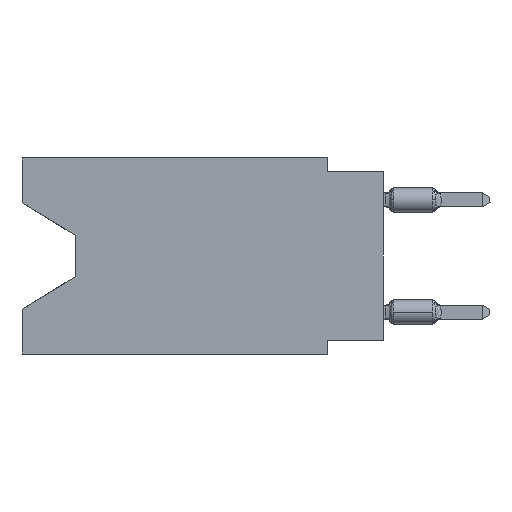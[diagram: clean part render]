
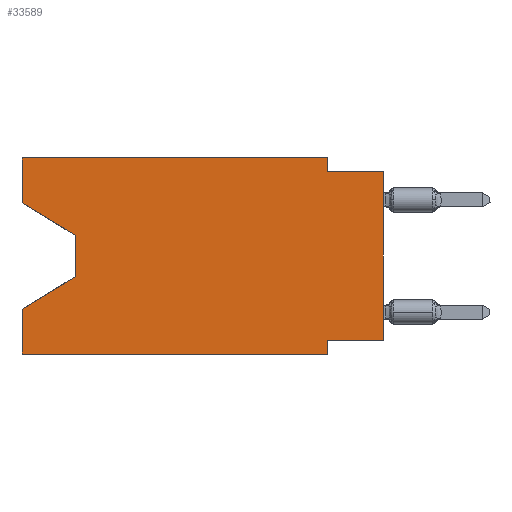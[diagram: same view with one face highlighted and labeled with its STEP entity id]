
A CAD part, left-side view. The second image highlights one B-rep face of the part: STEP entity #33589.
In plain terms, the highlighted planar face has unit normal (-1, 0, 0).
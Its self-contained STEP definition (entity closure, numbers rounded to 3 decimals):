
#683 = DIRECTION ( 'NONE',  ( 0., 0., 1. ) ) ;
#956 = CARTESIAN_POINT ( 'NONE',  ( 0., 2.54, -8.255 ) ) ;
#1462 = DIRECTION ( 'NONE',  ( 0., -0.855, -0.519 ) ) ;
#2571 = ORIENTED_EDGE ( 'NONE', *, *, #12025, .F. ) ;
#3016 = CARTESIAN_POINT ( 'NONE',  ( 0., 13.97, -5.385 ) ) ;
#3357 = EDGE_CURVE ( 'NONE', #35843, #12292, #34434, .T. ) ;
#3994 = LINE ( 'NONE', #14926, #8670 ) ;
#4325 = ORIENTED_EDGE ( 'NONE', *, *, #32457, .F. ) ;
#4568 = ORIENTED_EDGE ( 'NONE', *, *, #39529, .F. ) ;
#4733 = CARTESIAN_POINT ( 'NONE',  ( 0., 16.383, -6.852 ) ) ;
#4931 = VECTOR ( 'NONE', #32310, 1000. ) ;
#5075 = ORIENTED_EDGE ( 'NONE', *, *, #31634, .F. ) ;
#5593 = VERTEX_POINT ( 'NONE', #46168 ) ;
#6111 = LINE ( 'NONE', #3016, #12749 ) ;
#7310 = DIRECTION ( 'NONE',  ( 0., 1., 0. ) ) ;
#8323 = CARTESIAN_POINT ( 'NONE',  ( 0., 13.97, -3.505 ) ) ;
#8378 = DIRECTION ( 'NONE',  ( 0., -1., 0. ) ) ;
#8670 = VECTOR ( 'NONE', #683, 1000. ) ;
#8930 = EDGE_CURVE ( 'NONE', #29006, #25882, #6111, .T. ) ;
#9010 = VECTOR ( 'NONE', #12647, 1000. ) ;
#11980 = DIRECTION ( 'NONE',  ( 0., -1., 0. ) ) ;
#12025 = EDGE_CURVE ( 'NONE', #16454, #5593, #29225, .T. ) ;
#12292 = VERTEX_POINT ( 'NONE', #23740 ) ;
#12314 = CARTESIAN_POINT ( 'NONE',  ( 0., 13.97, -5.385 ) ) ;
#12479 = CARTESIAN_POINT ( 'NONE',  ( 0., 16.383, 0. ) ) ;
#12647 = DIRECTION ( 'NONE',  ( 0., 0., -1. ) ) ;
#12749 = VECTOR ( 'NONE', #20538, 1000. ) ;
#13089 = CARTESIAN_POINT ( 'NONE',  ( 0., 0., -8.255 ) ) ;
#13542 = EDGE_CURVE ( 'NONE', #32646, #16454, #29089, .T. ) ;
#13664 = ORIENTED_EDGE ( 'NONE', *, *, #8930, .T. ) ;
#14042 = VECTOR ( 'NONE', #8378, 1000. ) ;
#14347 = CARTESIAN_POINT ( 'NONE',  ( 0., 2.54, -8.89 ) ) ;
#14559 = EDGE_CURVE ( 'NONE', #20537, #5593, #26353, .T. ) ;
#14644 = LINE ( 'NONE', #29059, #44240 ) ;
#14926 = CARTESIAN_POINT ( 'NONE',  ( 0., 16.383, 0. ) ) ;
#15206 = LINE ( 'NONE', #8323, #23613 ) ;
#16454 = VERTEX_POINT ( 'NONE', #956 ) ;
#17372 = CARTESIAN_POINT ( 'NONE',  ( 0., 0., -8.255 ) ) ;
#17870 = LINE ( 'NONE', #40113, #4931 ) ;
#17963 = CARTESIAN_POINT ( 'NONE',  ( 0., 16.383, 0. ) ) ;
#19497 = CARTESIAN_POINT ( 'NONE',  ( 0., 2.54, 0. ) ) ;
#20196 = VECTOR ( 'NONE', #40579, 1000. ) ;
#20537 = VERTEX_POINT ( 'NONE', #46764 ) ;
#20538 = DIRECTION ( 'NONE',  ( 0., 0.855, -0.519 ) ) ;
#21754 = CARTESIAN_POINT ( 'NONE',  ( 0., 13.97, -3.505 ) ) ;
#22084 = ORIENTED_EDGE ( 'NONE', *, *, #40878, .F. ) ;
#22279 = LINE ( 'NONE', #22744, #36389 ) ;
#22744 = CARTESIAN_POINT ( 'NONE',  ( 0., 16.383, 0. ) ) ;
#23613 = VECTOR ( 'NONE', #34120, 1000. ) ;
#23740 = CARTESIAN_POINT ( 'NONE',  ( 0., 2.54, -0.635 ) ) ;
#24313 = ORIENTED_EDGE ( 'NONE', *, *, #13542, .F. ) ;
#25882 = VERTEX_POINT ( 'NONE', #4733 ) ;
#26216 = DIRECTION ( 'NONE',  ( 0., 0., -1. ) ) ;
#26319 = CARTESIAN_POINT ( 'NONE',  ( 0., 16.383, -2.038 ) ) ;
#26353 = LINE ( 'NONE', #40806, #14042 ) ;
#26596 = EDGE_LOOP ( 'NONE', ( #43565, #34264, #13664, #5075, #45835, #2571, #24313, #46116, #22084, #37100, #4325, #4568 ) ) ;
#27401 = VERTEX_POINT ( 'NONE', #21754 ) ;
#28870 = VERTEX_POINT ( 'NONE', #30532 ) ;
#29006 = VERTEX_POINT ( 'NONE', #12314 ) ;
#29059 = CARTESIAN_POINT ( 'NONE',  ( 0., 0., 0. ) ) ;
#29089 = LINE ( 'NONE', #13089, #41152 ) ;
#29225 = LINE ( 'NONE', #14347, #20196 ) ;
#30532 = CARTESIAN_POINT ( 'NONE',  ( 0., 16.383, -2.038 ) ) ;
#31600 = CARTESIAN_POINT ( 'NONE',  ( 0., 0., -0.635 ) ) ;
#31634 = EDGE_CURVE ( 'NONE', #20537, #25882, #3994, .T. ) ;
#32310 = DIRECTION ( 'NONE',  ( 0., -1., 0. ) ) ;
#32457 = EDGE_CURVE ( 'NONE', #37434, #35843, #17870, .T. ) ;
#32646 = VERTEX_POINT ( 'NONE', #17372 ) ;
#33589 = ADVANCED_FACE ( 'NONE', ( #43758 ), #44425, .F. ) ;
#33707 = CARTESIAN_POINT ( 'NONE',  ( 0., 2.54, 0. ) ) ;
#34120 = DIRECTION ( 'NONE',  ( 0., 0., -1. ) ) ;
#34264 = ORIENTED_EDGE ( 'NONE', *, *, #41236, .T. ) ;
#34434 = LINE ( 'NONE', #19497, #9010 ) ;
#35843 = VERTEX_POINT ( 'NONE', #33707 ) ;
#36389 = VECTOR ( 'NONE', #36725, 1000. ) ;
#36725 = DIRECTION ( 'NONE',  ( 0., 0., 1. ) ) ;
#36986 = EDGE_CURVE ( 'NONE', #28870, #27401, #41457, .T. ) ;
#37081 = LINE ( 'NONE', #44391, #45505 ) ;
#37100 = ORIENTED_EDGE ( 'NONE', *, *, #3357, .F. ) ;
#37434 = VERTEX_POINT ( 'NONE', #12479 ) ;
#38756 = VECTOR ( 'NONE', #1462, 1000. ) ;
#39529 = EDGE_CURVE ( 'NONE', #28870, #37434, #22279, .T. ) ;
#40113 = CARTESIAN_POINT ( 'NONE',  ( 0., 16.383, 0. ) ) ;
#40440 = DIRECTION ( 'NONE',  ( 1., 0., 0. ) ) ;
#40579 = DIRECTION ( 'NONE',  ( 0., 0., -1. ) ) ;
#40806 = CARTESIAN_POINT ( 'NONE',  ( 0., 16.383, -8.89 ) ) ;
#40878 = EDGE_CURVE ( 'NONE', #12292, #43611, #37081, .T. ) ;
#41152 = VECTOR ( 'NONE', #7310, 1000. ) ;
#41194 = AXIS2_PLACEMENT_3D ( 'NONE', #17963, #40440, #26216 ) ;
#41236 = EDGE_CURVE ( 'NONE', #27401, #29006, #15206, .T. ) ;
#41457 = LINE ( 'NONE', #26319, #38756 ) ;
#43502 = DIRECTION ( 'NONE',  ( 0., 0., 1. ) ) ;
#43565 = ORIENTED_EDGE ( 'NONE', *, *, #36986, .T. ) ;
#43611 = VERTEX_POINT ( 'NONE', #31600 ) ;
#43758 = FACE_OUTER_BOUND ( 'NONE', #26596, .T. ) ;
#44240 = VECTOR ( 'NONE', #43502, 1000. ) ;
#44391 = CARTESIAN_POINT ( 'NONE',  ( 0., 0., -0.635 ) ) ;
#44425 = PLANE ( 'NONE',  #41194 ) ;
#44773 = EDGE_CURVE ( 'NONE', #32646, #43611, #14644, .T. ) ;
#45505 = VECTOR ( 'NONE', #11980, 1000. ) ;
#45835 = ORIENTED_EDGE ( 'NONE', *, *, #14559, .T. ) ;
#46116 = ORIENTED_EDGE ( 'NONE', *, *, #44773, .T. ) ;
#46168 = CARTESIAN_POINT ( 'NONE',  ( 0., 2.54, -8.89 ) ) ;
#46764 = CARTESIAN_POINT ( 'NONE',  ( 0., 16.383, -8.89 ) ) ;
